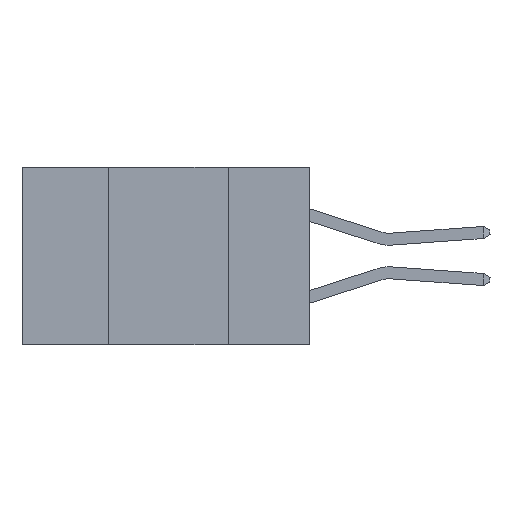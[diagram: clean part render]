
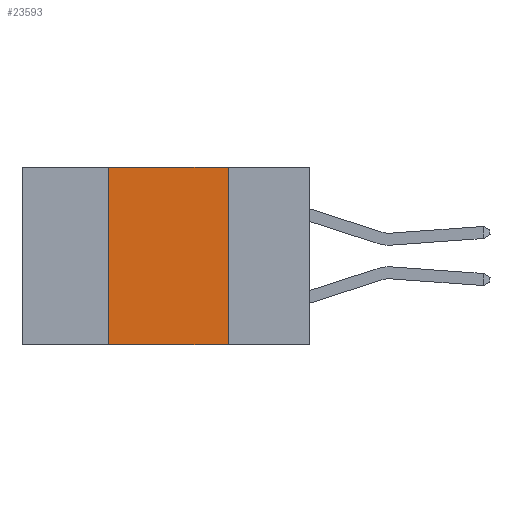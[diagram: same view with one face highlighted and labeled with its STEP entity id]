
A CAD part, left-side view. The second image highlights one B-rep face of the part: STEP entity #23593.
In plain terms, the highlighted planar face has unit normal (-1, 0, 0).
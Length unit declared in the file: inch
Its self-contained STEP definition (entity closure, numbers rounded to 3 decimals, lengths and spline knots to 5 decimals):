
#558 = EDGE_CURVE ( 'NONE', #869, #11877, #739, .T. ) ;
#739 = LINE ( 'NONE', #6492, #4301 ) ;
#810 = DIRECTION ( 'NONE',  ( 0., 0., 1. ) ) ;
#869 = VERTEX_POINT ( 'NONE', #21836 ) ;
#1390 = VERTEX_POINT ( 'NONE', #1962 ) ;
#1566 = ORIENTED_EDGE ( 'NONE', *, *, #12498, .F. ) ;
#1962 = CARTESIAN_POINT ( 'NONE',  ( 0., 0.42, 0. ) ) ;
#2471 = CARTESIAN_POINT ( 'NONE',  ( 0., 0.42, 0. ) ) ;
#4301 = VECTOR ( 'NONE', #15835, 39.37008 ) ;
#4730 = DIRECTION ( 'NONE',  ( 0., -1., 0. ) ) ;
#4914 = ORIENTED_EDGE ( 'NONE', *, *, #9460, .F. ) ;
#5095 = DIRECTION ( 'NONE',  ( 0., 0., -1. ) ) ;
#5306 = CARTESIAN_POINT ( 'NONE',  ( 0., 0.17, -0.37 ) ) ;
#5462 = LINE ( 'NONE', #14342, #6928 ) ;
#5575 = PLANE ( 'NONE',  #17600 ) ;
#5697 = LINE ( 'NONE', #14441, #8585 ) ;
#6492 = CARTESIAN_POINT ( 'NONE',  ( 0., 0.6, -0.37 ) ) ;
#6928 = VECTOR ( 'NONE', #4730, 39.37008 ) ;
#8585 = VECTOR ( 'NONE', #5095, 39.37008 ) ;
#9460 = EDGE_CURVE ( 'NONE', #869, #1390, #14337, .T. ) ;
#10327 = EDGE_CURVE ( 'NONE', #1390, #13098, #5462, .T. ) ;
#11207 = CARTESIAN_POINT ( 'NONE',  ( 0., 0.6, 0. ) ) ;
#11877 = VERTEX_POINT ( 'NONE', #5306 ) ;
#12498 = EDGE_CURVE ( 'NONE', #13098, #11877, #5697, .T. ) ;
#13078 = CARTESIAN_POINT ( 'NONE',  ( 0., 0.17, 0. ) ) ;
#13098 = VERTEX_POINT ( 'NONE', #13078 ) ;
#14337 = LINE ( 'NONE', #2471, #19031 ) ;
#14342 = CARTESIAN_POINT ( 'NONE',  ( 0., 0.6, 0. ) ) ;
#14441 = CARTESIAN_POINT ( 'NONE',  ( 0., 0.17, 0. ) ) ;
#14838 = DIRECTION ( 'NONE',  ( 1., 0., 0. ) ) ;
#15835 = DIRECTION ( 'NONE',  ( 0., -1., 0. ) ) ;
#16875 = ORIENTED_EDGE ( 'NONE', *, *, #558, .T. ) ;
#16987 = DIRECTION ( 'NONE',  ( 0., 0., -1. ) ) ;
#17600 = AXIS2_PLACEMENT_3D ( 'NONE', #11207, #14838, #16987 ) ;
#18855 = EDGE_LOOP ( 'NONE', ( #1566, #20181, #4914, #16875 ) ) ;
#19031 = VECTOR ( 'NONE', #810, 39.37008 ) ;
#19442 = FACE_OUTER_BOUND ( 'NONE', #18855, .T. ) ;
#20181 = ORIENTED_EDGE ( 'NONE', *, *, #10327, .F. ) ;
#21836 = CARTESIAN_POINT ( 'NONE',  ( 0., 0.42, -0.37 ) ) ;
#23593 = ADVANCED_FACE ( 'NONE', ( #19442 ), #5575, .F. ) ;
